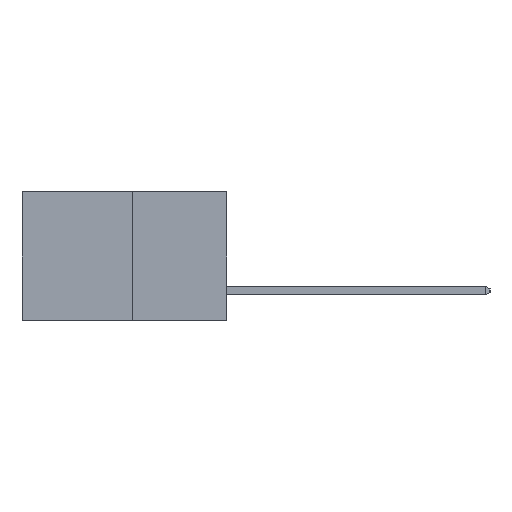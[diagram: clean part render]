
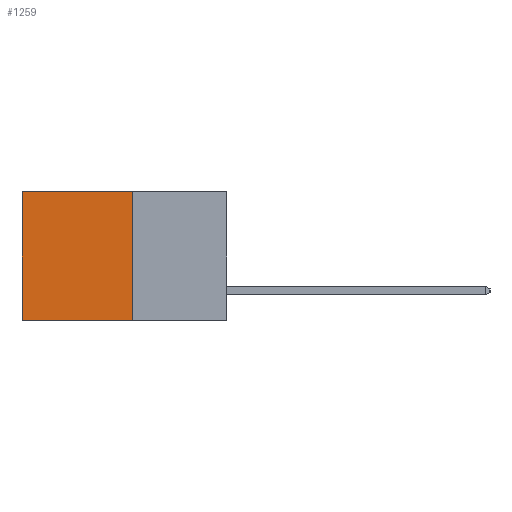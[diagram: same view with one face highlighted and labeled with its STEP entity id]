
A CAD part, left-side view. The second image highlights one B-rep face of the part: STEP entity #1259.
In plain terms, the highlighted planar face has unit normal (-1, 0, 0).
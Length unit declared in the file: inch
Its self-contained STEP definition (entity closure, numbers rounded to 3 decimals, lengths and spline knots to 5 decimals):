
#132 = VECTOR ( 'NONE', #5371, 39.37008 ) ;
#482 = VERTEX_POINT ( 'NONE', #4569 ) ;
#838 = DIRECTION ( 'NONE',  ( 0., 1., 0. ) ) ;
#886 = CARTESIAN_POINT ( 'NONE',  ( 0.277, 0.27, -0.37 ) ) ;
#1024 = LINE ( 'NONE', #9464, #9700 ) ;
#1250 = EDGE_CURVE ( 'NONE', #1334, #482, #1024, .T. ) ;
#1259 = ADVANCED_FACE ( 'NONE', ( #7261 ), #7563, .F. ) ;
#1334 = VERTEX_POINT ( 'NONE', #7194 ) ;
#1911 = VERTEX_POINT ( 'NONE', #2880 ) ;
#2274 = DIRECTION ( 'NONE',  ( 0., 1., 0. ) ) ;
#2529 = CARTESIAN_POINT ( 'NONE',  ( 0.277, 0.27, 0. ) ) ;
#2880 = CARTESIAN_POINT ( 'NONE',  ( 0.277, 0.59, 0. ) ) ;
#3577 = EDGE_CURVE ( 'NONE', #1911, #3926, #4650, .T. ) ;
#3926 = VERTEX_POINT ( 'NONE', #8275 ) ;
#4179 = LINE ( 'NONE', #2529, #6036 ) ;
#4569 = CARTESIAN_POINT ( 'NONE',  ( 0.277, 0.27, -0.37 ) ) ;
#4637 = EDGE_LOOP ( 'NONE', ( #6588, #7036, #5845, #8558 ) ) ;
#4650 = LINE ( 'NONE', #7532, #132 ) ;
#5164 = EDGE_CURVE ( 'NONE', #482, #3926, #6954, .T. ) ;
#5371 = DIRECTION ( 'NONE',  ( 0., 0., -1. ) ) ;
#5403 = CARTESIAN_POINT ( 'NONE',  ( 0.277, 0.27, -0.37 ) ) ;
#5459 = DIRECTION ( 'NONE',  ( 1., 0., 0. ) ) ;
#5845 = ORIENTED_EDGE ( 'NONE', *, *, #1250, .F. ) ;
#6036 = VECTOR ( 'NONE', #2274, 39.37008 ) ;
#6336 = EDGE_CURVE ( 'NONE', #1334, #1911, #4179, .T. ) ;
#6465 = AXIS2_PLACEMENT_3D ( 'NONE', #5403, #5459, #9723 ) ;
#6588 = ORIENTED_EDGE ( 'NONE', *, *, #3577, .T. ) ;
#6626 = DIRECTION ( 'NONE',  ( 0., 0., -1. ) ) ;
#6699 = VECTOR ( 'NONE', #838, 39.37008 ) ;
#6954 = LINE ( 'NONE', #886, #6699 ) ;
#7036 = ORIENTED_EDGE ( 'NONE', *, *, #5164, .F. ) ;
#7194 = CARTESIAN_POINT ( 'NONE',  ( 0.277, 0.27, 0. ) ) ;
#7261 = FACE_OUTER_BOUND ( 'NONE', #4637, .T. ) ;
#7532 = CARTESIAN_POINT ( 'NONE',  ( 0.277, 0.59, -0.37 ) ) ;
#7563 = PLANE ( 'NONE',  #6465 ) ;
#8275 = CARTESIAN_POINT ( 'NONE',  ( 0.277, 0.59, -0.37 ) ) ;
#8558 = ORIENTED_EDGE ( 'NONE', *, *, #6336, .T. ) ;
#9464 = CARTESIAN_POINT ( 'NONE',  ( 0.277, 0.27, -0.37 ) ) ;
#9700 = VECTOR ( 'NONE', #6626, 39.37008 ) ;
#9723 = DIRECTION ( 'NONE',  ( 0., 0., -1. ) ) ;
